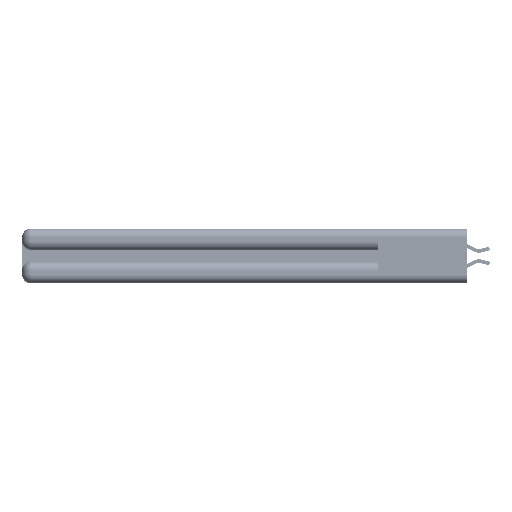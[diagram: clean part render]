
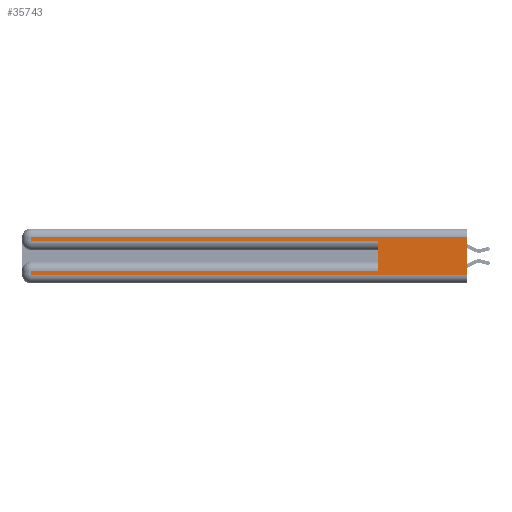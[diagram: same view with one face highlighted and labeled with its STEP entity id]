
A CAD part, left-side view. The second image highlights one B-rep face of the part: STEP entity #35743.
In plain terms, the highlighted planar face has unit normal (-1, 0, 0).
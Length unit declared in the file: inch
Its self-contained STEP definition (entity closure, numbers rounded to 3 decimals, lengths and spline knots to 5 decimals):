
#976 = EDGE_CURVE ( 'NONE', #50406, #49439, #3748, .T. ) ;
#1477 = ORIENTED_EDGE ( 'NONE', *, *, #53937, .T. ) ;
#2024 = VECTOR ( 'NONE', #52151, 39.37008 ) ;
#2360 = CARTESIAN_POINT ( 'NONE',  ( 0., 0.6, 0.085 ) ) ;
#3058 = CARTESIAN_POINT ( 'NONE',  ( 0., 0., 0.06 ) ) ;
#3113 = DIRECTION ( 'NONE',  ( 0., 0., -1. ) ) ;
#3748 = LINE ( 'NONE', #53569, #24886 ) ;
#4131 = ORIENTED_EDGE ( 'NONE', *, *, #976, .F. ) ;
#6003 = CARTESIAN_POINT ( 'NONE',  ( 0., 0., 0.31 ) ) ;
#7206 = LINE ( 'NONE', #54254, #17050 ) ;
#7918 = LINE ( 'NONE', #39714, #51384 ) ;
#9625 = DIRECTION ( 'NONE',  ( 1., 0., 0. ) ) ;
#12484 = DIRECTION ( 'NONE',  ( 0., 1., 0. ) ) ;
#12869 = DIRECTION ( 'NONE',  ( 0., -1., 0. ) ) ;
#13229 = LINE ( 'NONE', #35274, #2024 ) ;
#14415 = EDGE_CURVE ( 'NONE', #24543, #52930, #13229, .T. ) ;
#15471 = EDGE_CURVE ( 'NONE', #50574, #40285, #7918, .T. ) ;
#15515 = LINE ( 'NONE', #19814, #35357 ) ;
#16504 = CARTESIAN_POINT ( 'NONE',  ( 0., 2.94, 0.31 ) ) ;
#17050 = VECTOR ( 'NONE', #37619, 39.37008 ) ;
#18721 = AXIS2_PLACEMENT_3D ( 'NONE', #34926, #9625, #39193 ) ;
#19814 = CARTESIAN_POINT ( 'NONE',  ( 0., 0., 0.31 ) ) ;
#20058 = ORIENTED_EDGE ( 'NONE', *, *, #49399, .T. ) ;
#20394 = CARTESIAN_POINT ( 'NONE',  ( 0., 2.94, 0.285 ) ) ;
#20508 = FACE_OUTER_BOUND ( 'NONE', #36657, .T. ) ;
#20648 = ORIENTED_EDGE ( 'NONE', *, *, #38894, .T. ) ;
#22014 = ORIENTED_EDGE ( 'NONE', *, *, #14415, .F. ) ;
#24543 = VERTEX_POINT ( 'NONE', #2360 ) ;
#24886 = VECTOR ( 'NONE', #3113, 39.37008 ) ;
#25359 = ORIENTED_EDGE ( 'NONE', *, *, #15471, .T. ) ;
#25857 = VECTOR ( 'NONE', #12484, 39.37008 ) ;
#26419 = CARTESIAN_POINT ( 'NONE',  ( 0., 0.6, 0.285 ) ) ;
#27180 = DIRECTION ( 'NONE',  ( 0., 0., -1. ) ) ;
#27744 = VECTOR ( 'NONE', #28377, 39.37008 ) ;
#28377 = DIRECTION ( 'NONE',  ( 0., -1., 0. ) ) ;
#28635 = EDGE_CURVE ( 'NONE', #30815, #52930, #49674, .T. ) ;
#29337 = CARTESIAN_POINT ( 'NONE',  ( 0., 0., 0.085 ) ) ;
#30673 = PLANE ( 'NONE',  #18721 ) ;
#30705 = EDGE_CURVE ( 'NONE', #40285, #49439, #50077, .T. ) ;
#30815 = VERTEX_POINT ( 'NONE', #20394 ) ;
#33746 = CARTESIAN_POINT ( 'NONE',  ( 0., 0., 0.06 ) ) ;
#34926 = CARTESIAN_POINT ( 'NONE',  ( 0., 0., 0.37 ) ) ;
#35211 = ORIENTED_EDGE ( 'NONE', *, *, #28635, .T. ) ;
#35274 = CARTESIAN_POINT ( 'NONE',  ( 0., 0.6, 0.145 ) ) ;
#35357 = VECTOR ( 'NONE', #45082, 39.37008 ) ;
#35743 = ADVANCED_FACE ( 'NONE', ( #20508 ), #30673, .F. ) ;
#36657 = EDGE_LOOP ( 'NONE', ( #4131, #20648, #1477, #35211, #22014, #20058, #25359, #47772 ) ) ;
#37619 = DIRECTION ( 'NONE',  ( 0., 0., -1. ) ) ;
#38536 = VECTOR ( 'NONE', #12869, 39.37008 ) ;
#38894 = EDGE_CURVE ( 'NONE', #50406, #42249, #15515, .T. ) ;
#39193 = DIRECTION ( 'NONE',  ( 0., 0., -1. ) ) ;
#39714 = CARTESIAN_POINT ( 'NONE',  ( 0., 2.94, 0.37 ) ) ;
#40285 = VERTEX_POINT ( 'NONE', #52871 ) ;
#40659 = CARTESIAN_POINT ( 'NONE',  ( 0., 2.94, 0.085 ) ) ;
#42249 = VERTEX_POINT ( 'NONE', #16504 ) ;
#45082 = DIRECTION ( 'NONE',  ( 0., 1., 0. ) ) ;
#47772 = ORIENTED_EDGE ( 'NONE', *, *, #30705, .T. ) ;
#49399 = EDGE_CURVE ( 'NONE', #24543, #50574, #52189, .T. ) ;
#49439 = VERTEX_POINT ( 'NONE', #33746 ) ;
#49674 = LINE ( 'NONE', #50664, #38536 ) ;
#50077 = LINE ( 'NONE', #3058, #27744 ) ;
#50406 = VERTEX_POINT ( 'NONE', #6003 ) ;
#50574 = VERTEX_POINT ( 'NONE', #40659 ) ;
#50664 = CARTESIAN_POINT ( 'NONE',  ( 0., 0., 0.285 ) ) ;
#51384 = VECTOR ( 'NONE', #27180, 39.37008 ) ;
#52151 = DIRECTION ( 'NONE',  ( 0., 0., 1. ) ) ;
#52189 = LINE ( 'NONE', #29337, #25857 ) ;
#52871 = CARTESIAN_POINT ( 'NONE',  ( 0., 2.94, 0.06 ) ) ;
#52930 = VERTEX_POINT ( 'NONE', #26419 ) ;
#53569 = CARTESIAN_POINT ( 'NONE',  ( 0., 0., 0.37 ) ) ;
#53937 = EDGE_CURVE ( 'NONE', #42249, #30815, #7206, .T. ) ;
#54254 = CARTESIAN_POINT ( 'NONE',  ( 0., 2.94, 0.37 ) ) ;
